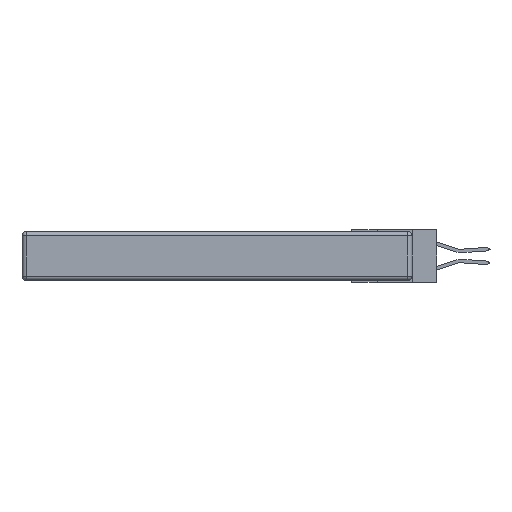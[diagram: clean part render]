
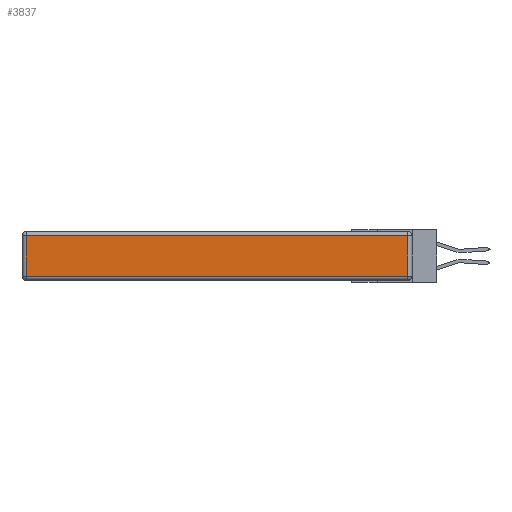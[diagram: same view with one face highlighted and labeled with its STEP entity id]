
A CAD part, left-side view. The second image highlights one B-rep face of the part: STEP entity #3837.
In plain terms, the highlighted planar face has unit normal (-1, 0, 0).
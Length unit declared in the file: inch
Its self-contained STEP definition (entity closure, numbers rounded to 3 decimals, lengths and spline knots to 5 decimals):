
#1495 = VECTOR ( 'NONE', #2683, 39.37008 ) ;
#1813 = LINE ( 'NONE', #10540, #8219 ) ;
#1997 = DIRECTION ( 'NONE',  ( 0., 0., -1. ) ) ;
#2171 = VERTEX_POINT ( 'NONE', #5494 ) ;
#2683 = DIRECTION ( 'NONE',  ( 0., -1., 0. ) ) ;
#3010 = EDGE_CURVE ( 'NONE', #4304, #6217, #7289, .T. ) ;
#3026 = ORIENTED_EDGE ( 'NONE', *, *, #11021, .T. ) ;
#3837 = ADVANCED_FACE ( 'NONE', ( #11666 ), #6640, .T. ) ;
#3881 = VECTOR ( 'NONE', #7353, 39.37008 ) ;
#4304 = VERTEX_POINT ( 'NONE', #6312 ) ;
#4417 = EDGE_CURVE ( 'NONE', #2171, #4304, #1813, .T. ) ;
#4490 = EDGE_CURVE ( 'NONE', #6801, #2171, #9624, .T. ) ;
#4979 = VECTOR ( 'NONE', #1997, 39.37008 ) ;
#5176 = EDGE_LOOP ( 'NONE', ( #7586, #6899, #10559, #3026 ) ) ;
#5277 = LINE ( 'NONE', #9028, #4979 ) ;
#5494 = CARTESIAN_POINT ( 'NONE',  ( 0., 0.03, -0.313 ) ) ;
#5543 = CARTESIAN_POINT ( 'NONE',  ( 0., 0., -0.313 ) ) ;
#5563 = DIRECTION ( 'NONE',  ( 0., 0., 1. ) ) ;
#6217 = VERTEX_POINT ( 'NONE', #11392 ) ;
#6312 = CARTESIAN_POINT ( 'NONE',  ( 0., 0.03, -0.03 ) ) ;
#6569 = CARTESIAN_POINT ( 'NONE',  ( 0., 2.72, -0.313 ) ) ;
#6640 = PLANE ( 'NONE',  #8786 ) ;
#6801 = VERTEX_POINT ( 'NONE', #6569 ) ;
#6899 = ORIENTED_EDGE ( 'NONE', *, *, #4417, .T. ) ;
#7289 = LINE ( 'NONE', #8223, #3881 ) ;
#7353 = DIRECTION ( 'NONE',  ( 0., 1., 0. ) ) ;
#7586 = ORIENTED_EDGE ( 'NONE', *, *, #4490, .T. ) ;
#8219 = VECTOR ( 'NONE', #8750, 39.37008 ) ;
#8223 = CARTESIAN_POINT ( 'NONE',  ( 0., 2.75, -0.03 ) ) ;
#8678 = CARTESIAN_POINT ( 'NONE',  ( 0., 0., -0.343 ) ) ;
#8750 = DIRECTION ( 'NONE',  ( 0., 0., 1. ) ) ;
#8786 = AXIS2_PLACEMENT_3D ( 'NONE', #8678, #12491, #5563 ) ;
#9028 = CARTESIAN_POINT ( 'NONE',  ( 0., 2.72, -0.343 ) ) ;
#9624 = LINE ( 'NONE', #5543, #1495 ) ;
#10540 = CARTESIAN_POINT ( 'NONE',  ( 0., 0.03, -0.343 ) ) ;
#10559 = ORIENTED_EDGE ( 'NONE', *, *, #3010, .T. ) ;
#11021 = EDGE_CURVE ( 'NONE', #6217, #6801, #5277, .T. ) ;
#11392 = CARTESIAN_POINT ( 'NONE',  ( 0., 2.72, -0.03 ) ) ;
#11666 = FACE_OUTER_BOUND ( 'NONE', #5176, .T. ) ;
#12491 = DIRECTION ( 'NONE',  ( -1., 0., 0. ) ) ;
